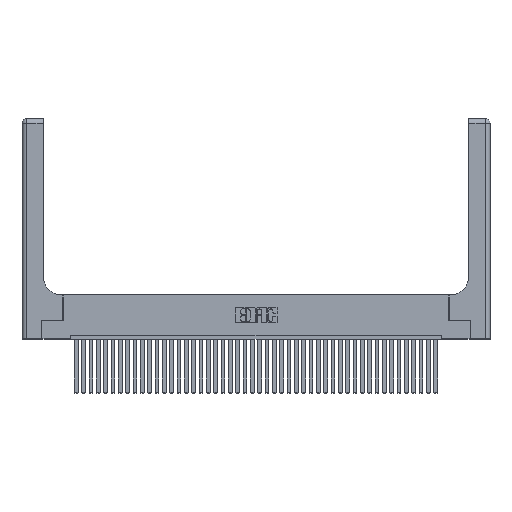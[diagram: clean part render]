
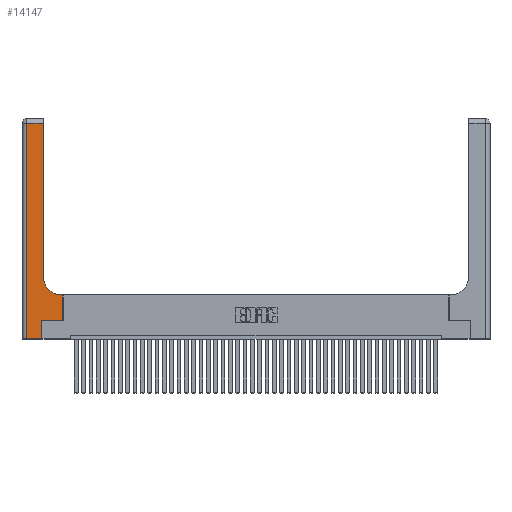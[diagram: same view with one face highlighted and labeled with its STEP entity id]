
A CAD part, top view. The second image highlights one B-rep face of the part: STEP entity #14147.
In plain terms, the highlighted planar face has unit normal (0, 0, 1).
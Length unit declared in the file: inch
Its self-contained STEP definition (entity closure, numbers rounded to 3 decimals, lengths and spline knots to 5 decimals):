
#457 = VERTEX_POINT ( 'NONE', #41490 ) ;
#1065 = VERTEX_POINT ( 'NONE', #25645 ) ;
#1342 = DIRECTION ( 'NONE',  ( -1., 0., 0. ) ) ;
#1345 = DIRECTION ( 'NONE',  ( 1., 0., 0. ) ) ;
#1798 = CARTESIAN_POINT ( 'NONE',  ( 0.06, 2.94, 0.37 ) ) ;
#3106 = EDGE_CURVE ( 'NONE', #24137, #1065, #23960, .T. ) ;
#3331 = DIRECTION ( 'NONE',  ( -1., 0., 0. ) ) ;
#3369 = AXIS2_PLACEMENT_3D ( 'NONE', #26998, #20853, #8055 ) ;
#3488 = ORIENTED_EDGE ( 'NONE', *, *, #21855, .T. ) ;
#3506 = LINE ( 'NONE', #10344, #31582 ) ;
#4012 = LINE ( 'NONE', #10717, #35530 ) ;
#4143 = PLANE ( 'NONE',  #35859 ) ;
#4439 = CARTESIAN_POINT ( 'NONE',  ( 0.2915, 0.6, 0.37 ) ) ;
#4592 = CARTESIAN_POINT ( 'NONE',  ( 0.269, 0.25, 0.37 ) ) ;
#4853 = EDGE_CURVE ( 'NONE', #9723, #7584, #16795, .T. ) ;
#5735 = CARTESIAN_POINT ( 'NONE',  ( 0., 0., 0.37 ) ) ;
#5966 = CARTESIAN_POINT ( 'NONE',  ( 0.5585, 0.25, 0.37 ) ) ;
#6590 = ORIENTED_EDGE ( 'NONE', *, *, #20233, .T. ) ;
#7381 = CARTESIAN_POINT ( 'NONE',  ( 0., 3., 0.37 ) ) ;
#7426 = CARTESIAN_POINT ( 'NONE',  ( 0.06, 0., 0.37 ) ) ;
#7584 = VERTEX_POINT ( 'NONE', #17126 ) ;
#7737 = EDGE_CURVE ( 'NONE', #29877, #457, #11081, .T. ) ;
#8055 = DIRECTION ( 'NONE',  ( 1., 0., 0. ) ) ;
#8423 = ORIENTED_EDGE ( 'NONE', *, *, #26157, .T. ) ;
#8666 = ORIENTED_EDGE ( 'NONE', *, *, #17415, .T. ) ;
#9536 = CARTESIAN_POINT ( 'NONE',  ( 0.2915, 3., 0.37 ) ) ;
#9723 = VERTEX_POINT ( 'NONE', #39104 ) ;
#9974 = VERTEX_POINT ( 'NONE', #1798 ) ;
#10052 = EDGE_CURVE ( 'NONE', #7584, #24137, #41055, .T. ) ;
#10344 = CARTESIAN_POINT ( 'NONE',  ( 0.269, 0., 0.37 ) ) ;
#10717 = CARTESIAN_POINT ( 'NONE',  ( 0.06, 3., 0.37 ) ) ;
#10785 = ORIENTED_EDGE ( 'NONE', *, *, #10052, .T. ) ;
#10984 = CARTESIAN_POINT ( 'NONE',  ( 0.269, 0.25, 0.37 ) ) ;
#11081 = LINE ( 'NONE', #5735, #22099 ) ;
#11193 = VERTEX_POINT ( 'NONE', #5966 ) ;
#11608 = ORIENTED_EDGE ( 'NONE', *, *, #3106, .T. ) ;
#12112 = VECTOR ( 'NONE', #39688, 39.37008 ) ;
#14147 = ADVANCED_FACE ( 'NONE', ( #27930 ), #4143, .F. ) ;
#14549 = ORIENTED_EDGE ( 'NONE', *, *, #4853, .T. ) ;
#16340 = DIRECTION ( 'NONE',  ( 1., 0., 0. ) ) ;
#16795 = LINE ( 'NONE', #4439, #20852 ) ;
#17126 = CARTESIAN_POINT ( 'NONE',  ( 0.5415, 0.6, 0.37 ) ) ;
#17198 = CARTESIAN_POINT ( 'NONE',  ( 0.5585, 0.25, 0.37 ) ) ;
#17415 = EDGE_CURVE ( 'NONE', #11193, #9723, #41239, .T. ) ;
#19954 = CARTESIAN_POINT ( 'NONE',  ( 0.2915, 0.85, 0.37 ) ) ;
#20233 = EDGE_CURVE ( 'NONE', #457, #25450, #3506, .T. ) ;
#20852 = VECTOR ( 'NONE', #1342, 39.37008 ) ;
#20853 = DIRECTION ( 'NONE',  ( 0., 0., -1. ) ) ;
#21397 = VECTOR ( 'NONE', #1345, 39.37008 ) ;
#21854 = VECTOR ( 'NONE', #3331, 39.37008 ) ;
#21855 = EDGE_CURVE ( 'NONE', #25450, #11193, #33949, .T. ) ;
#22099 = VECTOR ( 'NONE', #16340, 39.37008 ) ;
#23395 = DIRECTION ( 'NONE',  ( 0., 0., -1. ) ) ;
#23960 = LINE ( 'NONE', #9536, #38995 ) ;
#24137 = VERTEX_POINT ( 'NONE', #19954 ) ;
#25450 = VERTEX_POINT ( 'NONE', #10984 ) ;
#25645 = CARTESIAN_POINT ( 'NONE',  ( 0.2915, 2.94, 0.37 ) ) ;
#25917 = EDGE_CURVE ( 'NONE', #1065, #9974, #39379, .T. ) ;
#26157 = EDGE_CURVE ( 'NONE', #9974, #29877, #4012, .T. ) ;
#26998 = CARTESIAN_POINT ( 'NONE',  ( 0.5415, 0.85, 0.37 ) ) ;
#27930 = FACE_OUTER_BOUND ( 'NONE', #32369, .T. ) ;
#28055 = ORIENTED_EDGE ( 'NONE', *, *, #7737, .T. ) ;
#29446 = DIRECTION ( 'NONE',  ( 0., -1., 0. ) ) ;
#29877 = VERTEX_POINT ( 'NONE', #7426 ) ;
#31582 = VECTOR ( 'NONE', #36088, 39.37008 ) ;
#32005 = CARTESIAN_POINT ( 'NONE',  ( 0., 2.94, 0.37 ) ) ;
#32369 = EDGE_LOOP ( 'NONE', ( #11608, #37795, #8423, #28055, #6590, #3488, #8666, #14549, #10785 ) ) ;
#33071 = DIRECTION ( 'NONE',  ( -1., 0., 0. ) ) ;
#33949 = LINE ( 'NONE', #4592, #21397 ) ;
#35530 = VECTOR ( 'NONE', #29446, 39.37008 ) ;
#35859 = AXIS2_PLACEMENT_3D ( 'NONE', #7381, #23395, #33071 ) ;
#36088 = DIRECTION ( 'NONE',  ( 0., 1., 0. ) ) ;
#36942 = DIRECTION ( 'NONE',  ( 0., 1., 0. ) ) ;
#37795 = ORIENTED_EDGE ( 'NONE', *, *, #25917, .T. ) ;
#38995 = VECTOR ( 'NONE', #36942, 39.37008 ) ;
#39104 = CARTESIAN_POINT ( 'NONE',  ( 0.5585, 0.6, 0.37 ) ) ;
#39379 = LINE ( 'NONE', #32005, #21854 ) ;
#39688 = DIRECTION ( 'NONE',  ( 0., 1., 0. ) ) ;
#41055 = CIRCLE ( 'NONE', #3369, 0.25 ) ;
#41239 = LINE ( 'NONE', #17198, #12112 ) ;
#41490 = CARTESIAN_POINT ( 'NONE',  ( 0.269, 0., 0.37 ) ) ;
